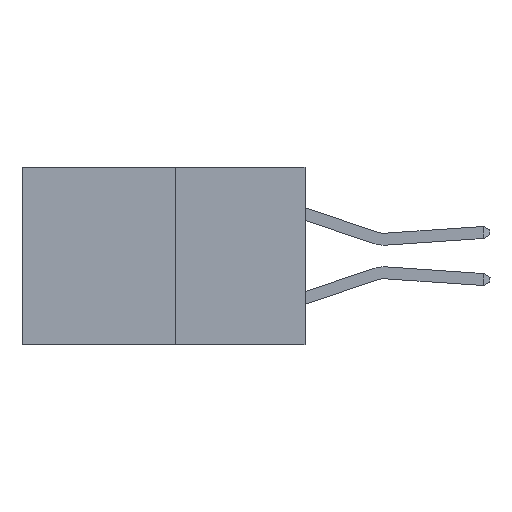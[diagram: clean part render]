
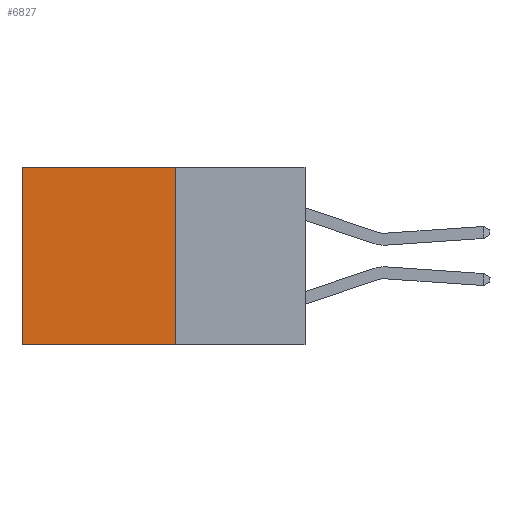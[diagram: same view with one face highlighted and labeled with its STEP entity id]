
A CAD part, left-side view. The second image highlights one B-rep face of the part: STEP entity #6827.
In plain terms, the highlighted planar face has unit normal (-1, 0, 0).
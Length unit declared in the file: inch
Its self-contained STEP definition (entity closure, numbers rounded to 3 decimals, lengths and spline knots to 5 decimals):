
#286 = VECTOR ( 'NONE', #9934, 39.37008 ) ;
#964 = LINE ( 'NONE', #5826, #14002 ) ;
#1026 = CARTESIAN_POINT ( 'NONE',  ( 0.277, 0.27, -0.37 ) ) ;
#1302 = FACE_OUTER_BOUND ( 'NONE', #12897, .T. ) ;
#1594 = CARTESIAN_POINT ( 'NONE',  ( 0.277, 0.27, -0.37 ) ) ;
#1929 = ORIENTED_EDGE ( 'NONE', *, *, #15323, .F. ) ;
#3034 = CARTESIAN_POINT ( 'NONE',  ( 0.277, 0.59, -0.37 ) ) ;
#3096 = VECTOR ( 'NONE', #7135, 39.37008 ) ;
#3207 = VERTEX_POINT ( 'NONE', #15920 ) ;
#4172 = DIRECTION ( 'NONE',  ( 0., 0., -1. ) ) ;
#4668 = EDGE_CURVE ( 'NONE', #3207, #12977, #9325, .T. ) ;
#5826 = CARTESIAN_POINT ( 'NONE',  ( 0.277, 0.27, -0.37 ) ) ;
#6700 = PLANE ( 'NONE',  #9155 ) ;
#6827 = ADVANCED_FACE ( 'NONE', ( #1302 ), #6700, .F. ) ;
#7135 = DIRECTION ( 'NONE',  ( 0., 0., -1. ) ) ;
#9155 = AXIS2_PLACEMENT_3D ( 'NONE', #1594, #11712, #4172 ) ;
#9325 = LINE ( 'NONE', #12507, #15959 ) ;
#9934 = DIRECTION ( 'NONE',  ( 0., 1., 0. ) ) ;
#10278 = ORIENTED_EDGE ( 'NONE', *, *, #15171, .T. ) ;
#10875 = DIRECTION ( 'NONE',  ( 0., 0., -1. ) ) ;
#11712 = DIRECTION ( 'NONE',  ( 1., 0., 0. ) ) ;
#12062 = DIRECTION ( 'NONE',  ( 0., 1., 0. ) ) ;
#12507 = CARTESIAN_POINT ( 'NONE',  ( 0.277, 0.27, 0. ) ) ;
#12567 = EDGE_CURVE ( 'NONE', #3207, #15970, #964, .T. ) ;
#12762 = LINE ( 'NONE', #14596, #3096 ) ;
#12897 = EDGE_LOOP ( 'NONE', ( #10278, #1929, #15162, #15986 ) ) ;
#12977 = VERTEX_POINT ( 'NONE', #15265 ) ;
#13344 = LINE ( 'NONE', #1026, #286 ) ;
#13494 = CARTESIAN_POINT ( 'NONE',  ( 0.277, 0.27, -0.37 ) ) ;
#14002 = VECTOR ( 'NONE', #10875, 39.37008 ) ;
#14596 = CARTESIAN_POINT ( 'NONE',  ( 0.277, 0.59, -0.37 ) ) ;
#15162 = ORIENTED_EDGE ( 'NONE', *, *, #12567, .F. ) ;
#15171 = EDGE_CURVE ( 'NONE', #12977, #15782, #12762, .T. ) ;
#15265 = CARTESIAN_POINT ( 'NONE',  ( 0.277, 0.59, 0. ) ) ;
#15323 = EDGE_CURVE ( 'NONE', #15970, #15782, #13344, .T. ) ;
#15782 = VERTEX_POINT ( 'NONE', #3034 ) ;
#15920 = CARTESIAN_POINT ( 'NONE',  ( 0.277, 0.27, 0. ) ) ;
#15959 = VECTOR ( 'NONE', #12062, 39.37008 ) ;
#15970 = VERTEX_POINT ( 'NONE', #13494 ) ;
#15986 = ORIENTED_EDGE ( 'NONE', *, *, #4668, .T. ) ;
